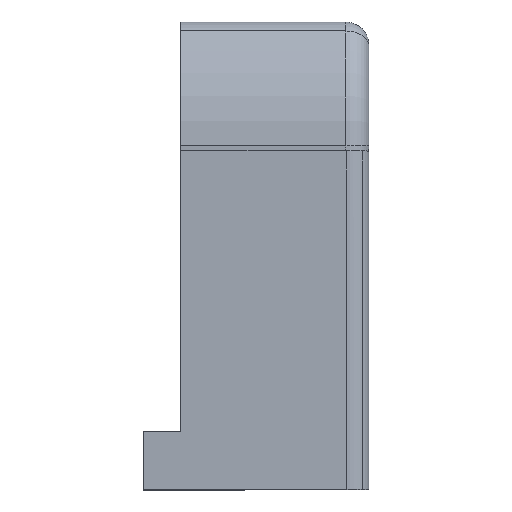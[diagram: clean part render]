
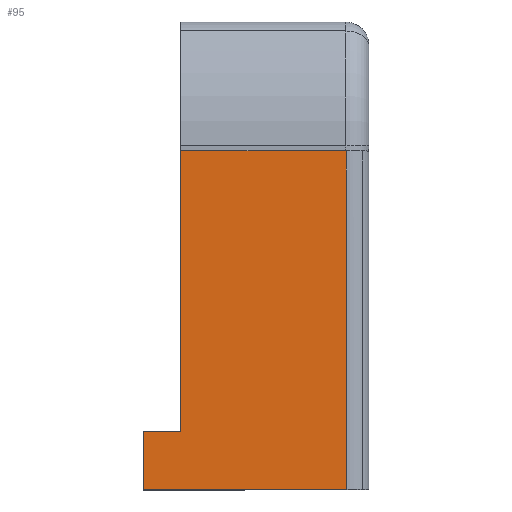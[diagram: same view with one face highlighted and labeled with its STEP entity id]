
A CAD part, top view. The second image highlights one B-rep face of the part: STEP entity #95.
In plain terms, the highlighted planar face has unit normal (0, 0, 1).
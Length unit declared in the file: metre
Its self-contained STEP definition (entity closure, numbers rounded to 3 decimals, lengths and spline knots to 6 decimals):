
#95=ADVANCED_FACE('0:2550',(#206),#207,.T.);
#206=FACE_OUTER_BOUND('',#326,.T.);
#207=PLANE('',#327);
#326=EDGE_LOOP('',(#725,#726,#727,#728,#729,#730));
#327=AXIS2_PLACEMENT_3D('',#731,#732,#733);
#725=ORIENTED_EDGE('',*,*,#902,.F.);
#726=ORIENTED_EDGE('',*,*,#882,.T.);
#727=ORIENTED_EDGE('',*,*,#925,.F.);
#728=ORIENTED_EDGE('',*,*,#932,.F.);
#729=ORIENTED_EDGE('',*,*,#933,.T.);
#730=ORIENTED_EDGE('',*,*,#928,.F.);
#731=CARTESIAN_POINT('',(0.032528,0.040065,0.018535));
#732=DIRECTION('',(0.0,0.,1.0));
#733=DIRECTION('',(0.0,-1.0,0.));
#882=EDGE_CURVE('0:2621',#1089,#1087,#1090,.T.);
#902=EDGE_CURVE('0:2708',#1089,#1116,#1117,.T.);
#925=EDGE_CURVE('0:2780',#1154,#1087,#1156,.T.);
#928=EDGE_CURVE('0:2789',#1116,#1160,#1161,.T.);
#932=EDGE_CURVE('0:2801',#1166,#1154,#1167,.T.);
#933=EDGE_CURVE('0:2804',#1166,#1160,#1168,.T.);
#1087=VERTEX_POINT('',#1347);
#1089=VERTEX_POINT('',#1349);
#1090=LINE('',#1350,#1351);
#1116=VERTEX_POINT('',#1382);
#1117=LINE('',#1383,#1384);
#1154=VERTEX_POINT('',#1439);
#1156=LINE('',#1442,#1443);
#1160=VERTEX_POINT('',#1449);
#1161=LINE('',#1450,#1451);
#1166=VERTEX_POINT('',#1459);
#1167=LINE('',#1460,#1461);
#1168=LINE('',#1462,#1463);
#1347=CARTESIAN_POINT('',(0.0119,0.036937,0.018534));
#1349=CARTESIAN_POINT('',(0.029961,0.036937,0.018534));
#1350=CARTESIAN_POINT('',(0.0117,0.036937,0.018533));
#1351=VECTOR('',#1688,1.0);
#1382=CARTESIAN_POINT('',(0.030011,0.00006,0.018535));
#1383=CARTESIAN_POINT('',(0.030011,0.030052,0.018535));
#1384=VECTOR('',#1736,1.0);
#1439=CARTESIAN_POINT('',(0.0119,0.00641,0.018535));
#1442=CARTESIAN_POINT('',(0.0119,0.028237,0.018535));
#1443=VECTOR('',#1765,1.0);
#1449=CARTESIAN_POINT('',(0.0078,0.00006,0.018535));
#1450=CARTESIAN_POINT('',(0.032528,0.00006,0.018535));
#1451=VECTOR('',#1768,1.0);
#1459=CARTESIAN_POINT('',(0.0078,0.00641,0.018535));
#1460=CARTESIAN_POINT('',(0.00535,0.00641,0.018535));
#1461=VECTOR('',#1772,1.0);
#1462=CARTESIAN_POINT('',(0.0078,0.023729,0.018535));
#1463=VECTOR('',#1773,1.0);
#1688=DIRECTION('',(-1.0,0.0,0.0));
#1736=DIRECTION('',(-0.0,-1.0,0.));
#1765=DIRECTION('',(0.0,1.0,0.));
#1768=DIRECTION('',(-1.0,0.0,0.0));
#1772=DIRECTION('',(1.0,0.0,0.0));
#1773=DIRECTION('',(0.0,-1.0,0.));
